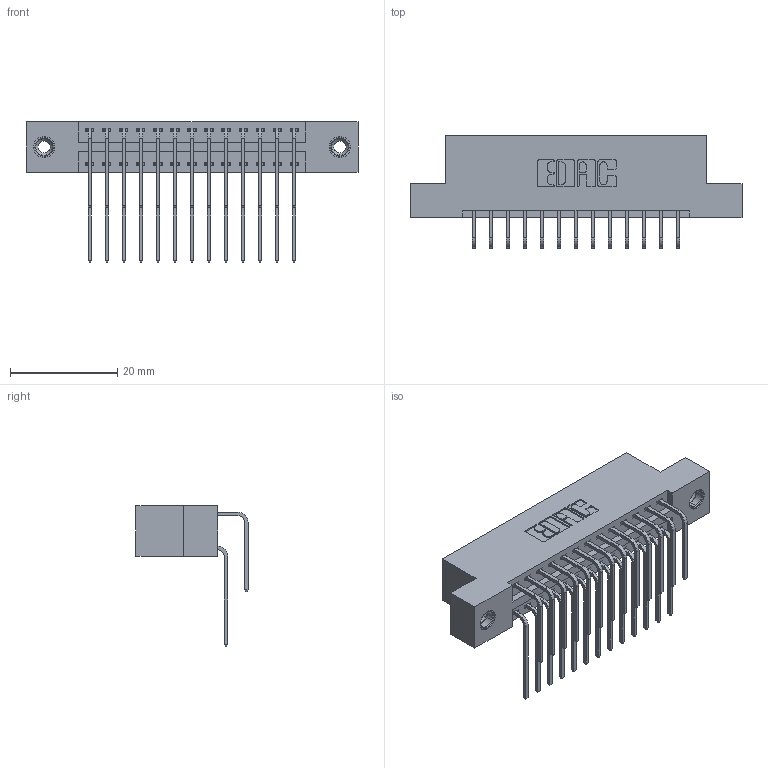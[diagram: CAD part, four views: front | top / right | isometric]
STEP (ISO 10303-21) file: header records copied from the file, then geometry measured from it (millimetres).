
FILE_DESCRIPTION (( 'STEP AP203' ), '1' );
FILE_NAME ('346-026-559-208.STEP', '2022-05-19T02:56:25', ( '' ), ( '' ), 'SwSTEP 2.0', 'SolidWorks 2020', '' );
FILE_SCHEMA (( 'CONFIG_CONTROL_DESIGN' ));
Length unit declared in the file: inch
Products named in the file (5): 345-292-001_559 Tail - 2; 345-292-001_558 559 Tail - 1; 346 Part_Flush Mounting Lugs - 0.156 Dia-TI; 345-250-001_345-250-003-102; 346-026-559-208
Assembly tree (29 placements, depth 2):
  346-026-559-208
    346 Part_Flush Mounting Lugs - 0.156 Dia-TI
    345-292-001_558 559 Tail - 1  x13
    345-292-001_559 Tail - 2  x13
    345-250-001_345-250-003-102  x2
Bounding box: 61.85 x 20.89 x 26.16 mm (x, y, z)
Volume: 5949.3 mm3; surface area: 8461.4 mm2
Topology: 29 solids, 29 shells, 1586 faces, 4651 edges, 3058 vertices
Faces by surface type: plane 1070, cylinder 500, cone 12, torus 4
Entity records: 15358 total; most frequent: CARTESIAN_POINT 2606, ORIENTED_EDGE 2482, DIRECTION 2347, EDGE_CURVE 1241, VECTOR 997, LINE 997, VERTEX_POINT 820, AXIS2_PLACEMENT_3D 675
